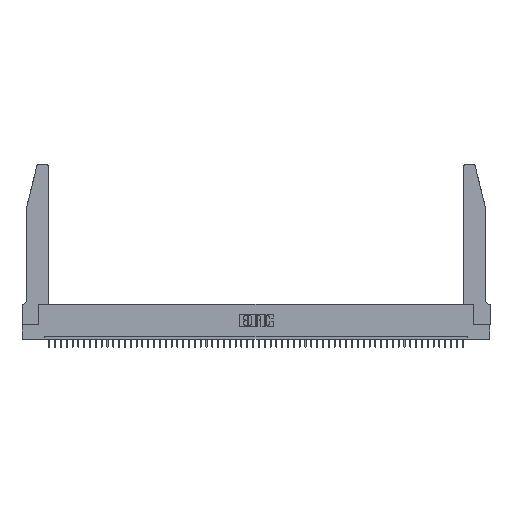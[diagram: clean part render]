
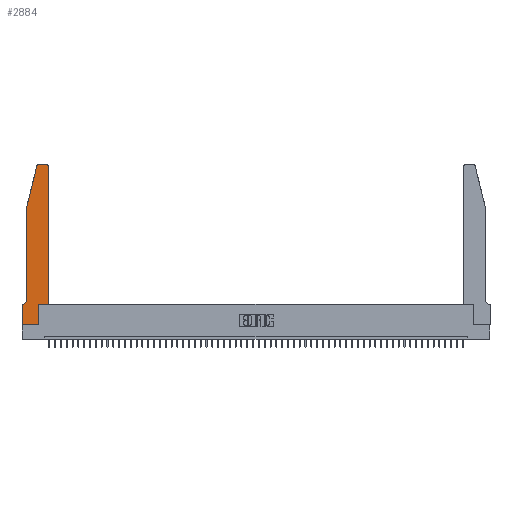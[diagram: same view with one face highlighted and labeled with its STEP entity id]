
A CAD part, top view. The second image highlights one B-rep face of the part: STEP entity #2884.
In plain terms, the highlighted planar face has unit normal (0, 0, 1).
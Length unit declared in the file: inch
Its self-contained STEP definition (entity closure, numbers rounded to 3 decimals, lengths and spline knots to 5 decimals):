
#64 = EDGE_CURVE ( 'NONE', #15971, #45576, #17803, .T. ) ;
#208 = DIRECTION ( 'NONE',  ( 0., 0., -1. ) ) ;
#1594 = CARTESIAN_POINT ( 'NONE',  ( 0.4505, 0.35, 0.37 ) ) ;
#2128 = ORIENTED_EDGE ( 'NONE', *, *, #48298, .T. ) ;
#2693 = DIRECTION ( 'NONE',  ( 0., 1., 0. ) ) ;
#2884 = ADVANCED_FACE ( 'NONE', ( #26794 ), #22063, .T. ) ;
#2891 = DIRECTION ( 'NONE',  ( -0.239, -0.971, 0. ) ) ;
#2980 = VECTOR ( 'NONE', #12392, 39.37008 ) ;
#3649 = VECTOR ( 'NONE', #31557, 39.37008 ) ;
#3807 = VECTOR ( 'NONE', #9448, 39.37008 ) ;
#3972 = VERTEX_POINT ( 'NONE', #7207 ) ;
#4367 = ORIENTED_EDGE ( 'NONE', *, *, #16116, .T. ) ;
#4442 = CARTESIAN_POINT ( 'NONE',  ( 0.0755, 2., 0.37 ) ) ;
#4612 = VERTEX_POINT ( 'NONE', #52935 ) ;
#5348 = AXIS2_PLACEMENT_3D ( 'NONE', #26387, #6337, #35278 ) ;
#5937 = LINE ( 'NONE', #14595, #3649 ) ;
#6337 = DIRECTION ( 'NONE',  ( 0., 0., 1. ) ) ;
#7190 = ORIENTED_EDGE ( 'NONE', *, *, #32877, .T. ) ;
#7207 = CARTESIAN_POINT ( 'NONE',  ( 0.0755, 0.42, 0.37 ) ) ;
#7355 = VECTOR ( 'NONE', #21448, 39.37008 ) ;
#8615 = CARTESIAN_POINT ( 'NONE',  ( 0.4505, 0.35, 0.37 ) ) ;
#8864 = CARTESIAN_POINT ( 'NONE',  ( 0.0055, 0.42, 0.37 ) ) ;
#9076 = VECTOR ( 'NONE', #2693, 39.37008 ) ;
#9448 = DIRECTION ( 'NONE',  ( 1., 0., 0. ) ) ;
#10023 = CARTESIAN_POINT ( 'NONE',  ( 0.2865, 0.35, 0.37 ) ) ;
#11267 = CARTESIAN_POINT ( 'NONE',  ( 0.0755, 2., 0.37 ) ) ;
#11338 = VECTOR ( 'NONE', #48422, 39.37008 ) ;
#11905 = VERTEX_POINT ( 'NONE', #16734 ) ;
#12392 = DIRECTION ( 'NONE',  ( -1., 0., 0. ) ) ;
#13767 = LINE ( 'NONE', #48255, #33909 ) ;
#14595 = CARTESIAN_POINT ( 'NONE',  ( 0.0755, 0.35, 0.37 ) ) ;
#15971 = VERTEX_POINT ( 'NONE', #33065 ) ;
#16116 = EDGE_CURVE ( 'NONE', #3972, #31370, #21453, .T. ) ;
#16376 = DIRECTION ( 'NONE',  ( 0., 0., 1. ) ) ;
#16734 = CARTESIAN_POINT ( 'NONE',  ( 0.4505, 2.72, 0.37 ) ) ;
#17803 = CIRCLE ( 'NONE', #5348, 0.03 ) ;
#18485 = DIRECTION ( 'NONE',  ( 0., 1., 0. ) ) ;
#18727 = CARTESIAN_POINT ( 'NONE',  ( 0., 0.35, 0.37 ) ) ;
#20910 = CARTESIAN_POINT ( 'NONE',  ( 0., 0., 0.37 ) ) ;
#21243 = ORIENTED_EDGE ( 'NONE', *, *, #33528, .T. ) ;
#21448 = DIRECTION ( 'NONE',  ( 0., -1., 0. ) ) ;
#21453 = CIRCLE ( 'NONE', #53424, 0.07 ) ;
#22063 = PLANE ( 'NONE',  #39979 ) ;
#22937 = ORIENTED_EDGE ( 'NONE', *, *, #44562, .T. ) ;
#23121 = CARTESIAN_POINT ( 'NONE',  ( 0.4205, 2.75, 0.37 ) ) ;
#23961 = CARTESIAN_POINT ( 'NONE',  ( 0.4205, 2.72, 0.37 ) ) ;
#25347 = VERTEX_POINT ( 'NONE', #41523 ) ;
#26387 = CARTESIAN_POINT ( 'NONE',  ( 0.284, 2.72, 0.37 ) ) ;
#26794 = FACE_OUTER_BOUND ( 'NONE', #46808, .T. ) ;
#27351 = DIRECTION ( 'NONE',  ( 1., 0., 0. ) ) ;
#28082 = ORIENTED_EDGE ( 'NONE', *, *, #51110, .T. ) ;
#28284 = LINE ( 'NONE', #1594, #9076 ) ;
#29162 = DIRECTION ( 'NONE',  ( 1., 0., 0. ) ) ;
#29790 = LINE ( 'NONE', #4442, #7355 ) ;
#30282 = DIRECTION ( 'NONE',  ( -1., 0., 0. ) ) ;
#30811 = ORIENTED_EDGE ( 'NONE', *, *, #47515, .T. ) ;
#30863 = EDGE_CURVE ( 'NONE', #31370, #35313, #5937, .T. ) ;
#31370 = VERTEX_POINT ( 'NONE', #48180 ) ;
#31460 = CARTESIAN_POINT ( 'NONE',  ( 0., 0., 0.37 ) ) ;
#31557 = DIRECTION ( 'NONE',  ( -1., 0., 0. ) ) ;
#31566 = VERTEX_POINT ( 'NONE', #33657 ) ;
#31665 = VECTOR ( 'NONE', #42045, 39.37008 ) ;
#32877 = EDGE_CURVE ( 'NONE', #25347, #3972, #29790, .T. ) ;
#33065 = CARTESIAN_POINT ( 'NONE',  ( 0.284, 2.75, 0.37 ) ) ;
#33528 = EDGE_CURVE ( 'NONE', #41906, #11905, #28284, .T. ) ;
#33657 = CARTESIAN_POINT ( 'NONE',  ( 0., 0., 0.37 ) ) ;
#33909 = VECTOR ( 'NONE', #18485, 39.37008 ) ;
#34479 = ORIENTED_EDGE ( 'NONE', *, *, #37045, .T. ) ;
#35278 = DIRECTION ( 'NONE',  ( 1., 0., 0. ) ) ;
#35285 = ORIENTED_EDGE ( 'NONE', *, *, #64, .T. ) ;
#35313 = VERTEX_POINT ( 'NONE', #37290 ) ;
#35442 = VERTEX_POINT ( 'NONE', #10023 ) ;
#35670 = DIRECTION ( 'NONE',  ( 0., 0., 1. ) ) ;
#36170 = LINE ( 'NONE', #31460, #11338 ) ;
#37045 = EDGE_CURVE ( 'NONE', #11905, #45976, #43080, .T. ) ;
#37290 = CARTESIAN_POINT ( 'NONE',  ( 0., 0.35, 0.37 ) ) ;
#37691 = LINE ( 'NONE', #41588, #2980 ) ;
#39478 = LINE ( 'NONE', #8615, #3807 ) ;
#39602 = VECTOR ( 'NONE', #2891, 39.37008 ) ;
#39979 = AXIS2_PLACEMENT_3D ( 'NONE', #18727, #35670, #27351 ) ;
#40158 = ORIENTED_EDGE ( 'NONE', *, *, #51656, .T. ) ;
#41024 = LINE ( 'NONE', #11267, #39602 ) ;
#41489 = ORIENTED_EDGE ( 'NONE', *, *, #30863, .T. ) ;
#41523 = CARTESIAN_POINT ( 'NONE',  ( 0.0755, 2., 0.37 ) ) ;
#41588 = CARTESIAN_POINT ( 'NONE',  ( 0.2605, 2.75, 0.37 ) ) ;
#41906 = VERTEX_POINT ( 'NONE', #49940 ) ;
#42045 = DIRECTION ( 'NONE',  ( 0., -1., 0. ) ) ;
#42159 = CARTESIAN_POINT ( 'NONE',  ( 0.25487, 2.72718, 0.37 ) ) ;
#43080 = CIRCLE ( 'NONE', #45735, 0.03 ) ;
#43123 = LINE ( 'NONE', #20910, #31665 ) ;
#44562 = EDGE_CURVE ( 'NONE', #4612, #35442, #13767, .T. ) ;
#45576 = VERTEX_POINT ( 'NONE', #42159 ) ;
#45735 = AXIS2_PLACEMENT_3D ( 'NONE', #23961, #16376, #29162 ) ;
#45976 = VERTEX_POINT ( 'NONE', #23121 ) ;
#46808 = EDGE_LOOP ( 'NONE', ( #2128, #35285, #28082, #7190, #4367, #41489, #40158, #53252, #22937, #30811, #21243, #34479 ) ) ;
#47515 = EDGE_CURVE ( 'NONE', #35442, #41906, #39478, .T. ) ;
#48180 = CARTESIAN_POINT ( 'NONE',  ( 0.0055, 0.35, 0.37 ) ) ;
#48255 = CARTESIAN_POINT ( 'NONE',  ( 0.2865, 0.35, 0.37 ) ) ;
#48298 = EDGE_CURVE ( 'NONE', #45976, #15971, #37691, .T. ) ;
#48422 = DIRECTION ( 'NONE',  ( 1., 0., 0. ) ) ;
#49940 = CARTESIAN_POINT ( 'NONE',  ( 0.4505, 0.35, 0.37 ) ) ;
#51110 = EDGE_CURVE ( 'NONE', #45576, #25347, #41024, .T. ) ;
#51656 = EDGE_CURVE ( 'NONE', #35313, #31566, #43123, .T. ) ;
#52935 = CARTESIAN_POINT ( 'NONE',  ( 0.2865, 0., 0.37 ) ) ;
#53080 = EDGE_CURVE ( 'NONE', #31566, #4612, #36170, .T. ) ;
#53252 = ORIENTED_EDGE ( 'NONE', *, *, #53080, .T. ) ;
#53424 = AXIS2_PLACEMENT_3D ( 'NONE', #8864, #208, #30282 ) ;
